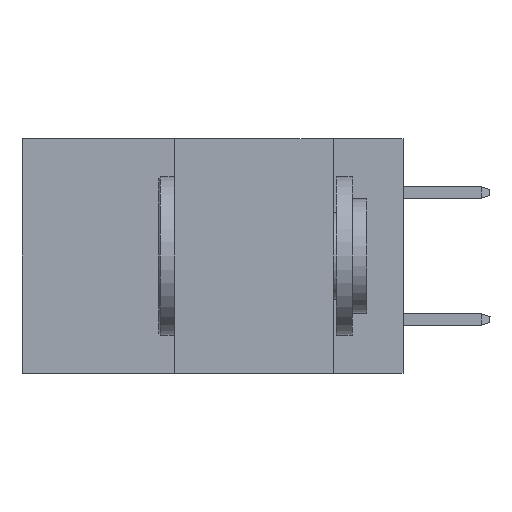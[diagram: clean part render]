
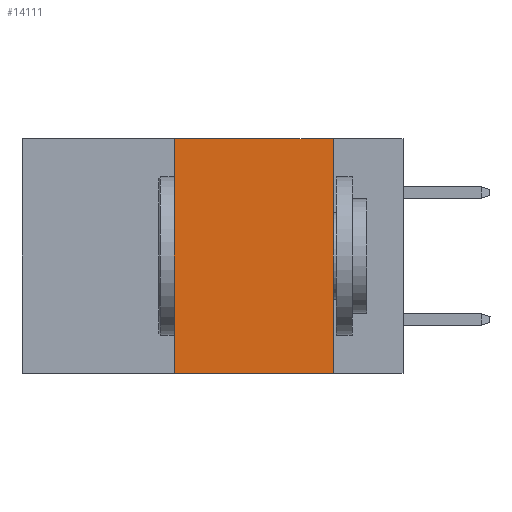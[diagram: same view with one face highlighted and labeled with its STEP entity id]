
A CAD part, left-side view. The second image highlights one B-rep face of the part: STEP entity #14111.
In plain terms, the highlighted planar face has unit normal (-1, 0, 0).
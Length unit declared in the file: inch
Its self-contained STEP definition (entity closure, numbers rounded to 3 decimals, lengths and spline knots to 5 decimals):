
#504 = AXIS2_PLACEMENT_3D ( 'NONE', #19845, #15562, #19694 ) ;
#2918 = LINE ( 'NONE', #20685, #20441 ) ;
#4346 = CARTESIAN_POINT ( 'NONE',  ( 0., 0.36, -0.37 ) ) ;
#4533 = VERTEX_POINT ( 'NONE', #23392 ) ;
#6151 = VERTEX_POINT ( 'NONE', #10058 ) ;
#6375 = DIRECTION ( 'NONE',  ( 0., 0., -1. ) ) ;
#6964 = VECTOR ( 'NONE', #23114, 39.37008 ) ;
#7716 = VERTEX_POINT ( 'NONE', #4346 ) ;
#8443 = CARTESIAN_POINT ( 'NONE',  ( 0., 0.11, 0. ) ) ;
#10058 = CARTESIAN_POINT ( 'NONE',  ( 0., 0.36, 0. ) ) ;
#11711 = LINE ( 'NONE', #20756, #6964 ) ;
#12278 = ORIENTED_EDGE ( 'NONE', *, *, #14112, .F. ) ;
#13984 = VERTEX_POINT ( 'NONE', #18569 ) ;
#14053 = ORIENTED_EDGE ( 'NONE', *, *, #22870, .F. ) ;
#14111 = ADVANCED_FACE ( 'NONE', ( #28782 ), #19991, .F. ) ;
#14112 = EDGE_CURVE ( 'NONE', #4533, #13984, #24600, .T. ) ;
#15039 = ORIENTED_EDGE ( 'NONE', *, *, #24574, .T. ) ;
#15562 = DIRECTION ( 'NONE',  ( 1., 0., 0. ) ) ;
#18569 = CARTESIAN_POINT ( 'NONE',  ( 0., 0.11, -0.37 ) ) ;
#18930 = VECTOR ( 'NONE', #6375, 39.37008 ) ;
#19694 = DIRECTION ( 'NONE',  ( 0., 0., -1. ) ) ;
#19845 = CARTESIAN_POINT ( 'NONE',  ( 0., 0.6, 0. ) ) ;
#19991 = PLANE ( 'NONE',  #504 ) ;
#20441 = VECTOR ( 'NONE', #25291, 39.37008 ) ;
#20685 = CARTESIAN_POINT ( 'NONE',  ( 0., 0.6, 0. ) ) ;
#20756 = CARTESIAN_POINT ( 'NONE',  ( 0., 0.36, 0. ) ) ;
#22205 = DIRECTION ( 'NONE',  ( 0., -1., 0. ) ) ;
#22264 = ORIENTED_EDGE ( 'NONE', *, *, #27582, .F. ) ;
#22506 = LINE ( 'NONE', #28914, #24587 ) ;
#22870 = EDGE_CURVE ( 'NONE', #7716, #6151, #11711, .T. ) ;
#23114 = DIRECTION ( 'NONE',  ( 0., 0., 1. ) ) ;
#23392 = CARTESIAN_POINT ( 'NONE',  ( 0., 0.11, 0. ) ) ;
#23414 = EDGE_LOOP ( 'NONE', ( #12278, #22264, #14053, #15039 ) ) ;
#24574 = EDGE_CURVE ( 'NONE', #7716, #13984, #22506, .T. ) ;
#24587 = VECTOR ( 'NONE', #22205, 39.37008 ) ;
#24600 = LINE ( 'NONE', #8443, #18930 ) ;
#25291 = DIRECTION ( 'NONE',  ( 0., -1., 0. ) ) ;
#27582 = EDGE_CURVE ( 'NONE', #6151, #4533, #2918, .T. ) ;
#28782 = FACE_OUTER_BOUND ( 'NONE', #23414, .T. ) ;
#28914 = CARTESIAN_POINT ( 'NONE',  ( 0., 0.6, -0.37 ) ) ;
